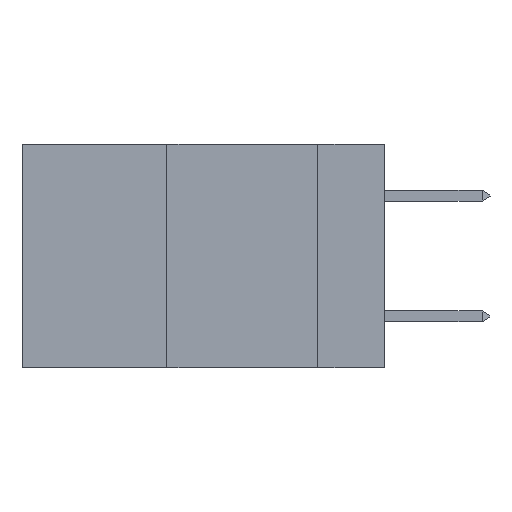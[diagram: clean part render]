
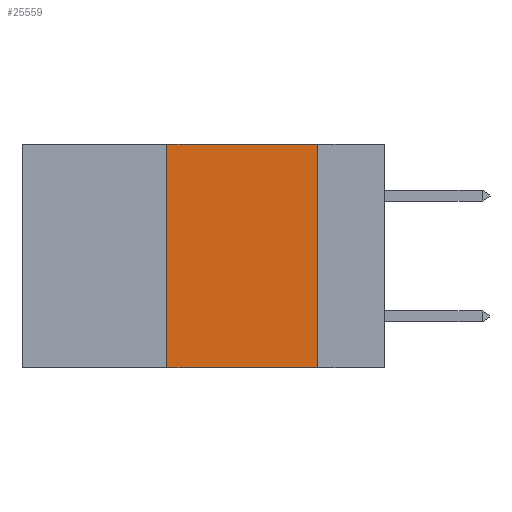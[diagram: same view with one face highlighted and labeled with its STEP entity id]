
A CAD part, left-side view. The second image highlights one B-rep face of the part: STEP entity #25559.
In plain terms, the highlighted planar face has unit normal (-1, 0, 0).
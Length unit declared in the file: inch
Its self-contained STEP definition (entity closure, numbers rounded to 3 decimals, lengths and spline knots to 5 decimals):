
#482 = CARTESIAN_POINT ( 'NONE',  ( 0., 0.6, 0. ) ) ;
#1963 = EDGE_LOOP ( 'NONE', ( #26776, #11105, #16997, #10084 ) ) ;
#3860 = LINE ( 'NONE', #15461, #24721 ) ;
#4085 = VERTEX_POINT ( 'NONE', #14336 ) ;
#4718 = DIRECTION ( 'NONE',  ( 0., 0., 1. ) ) ;
#6261 = LINE ( 'NONE', #32490, #35403 ) ;
#7123 = CARTESIAN_POINT ( 'NONE',  ( 0., 0.11, -0.37 ) ) ;
#7959 = CARTESIAN_POINT ( 'NONE',  ( 0., 0.6, 0. ) ) ;
#8156 = DIRECTION ( 'NONE',  ( 0., 0., -1. ) ) ;
#10084 = ORIENTED_EDGE ( 'NONE', *, *, #15928, .T. ) ;
#10442 = DIRECTION ( 'NONE',  ( 1., 0., 0. ) ) ;
#11105 = ORIENTED_EDGE ( 'NONE', *, *, #24320, .F. ) ;
#12488 = VECTOR ( 'NONE', #32417, 39.37008 ) ;
#13029 = VERTEX_POINT ( 'NONE', #32913 ) ;
#14336 = CARTESIAN_POINT ( 'NONE',  ( 0., 0.36, -0.37 ) ) ;
#15461 = CARTESIAN_POINT ( 'NONE',  ( 0., 0.11, 0. ) ) ;
#15928 = EDGE_CURVE ( 'NONE', #4085, #17012, #6261, .T. ) ;
#16038 = EDGE_CURVE ( 'NONE', #4085, #34879, #30956, .T. ) ;
#16997 = ORIENTED_EDGE ( 'NONE', *, *, #16038, .F. ) ;
#17012 = VERTEX_POINT ( 'NONE', #7123 ) ;
#19190 = FACE_OUTER_BOUND ( 'NONE', #1963, .T. ) ;
#21278 = CARTESIAN_POINT ( 'NONE',  ( 0., 0.36, 0. ) ) ;
#24134 = DIRECTION ( 'NONE',  ( 0., -1., 0. ) ) ;
#24320 = EDGE_CURVE ( 'NONE', #34879, #13029, #29759, .T. ) ;
#24721 = VECTOR ( 'NONE', #32192, 39.37008 ) ;
#25559 = ADVANCED_FACE ( 'NONE', ( #19190 ), #34376, .F. ) ;
#26229 = EDGE_CURVE ( 'NONE', #13029, #17012, #3860, .T. ) ;
#26776 = ORIENTED_EDGE ( 'NONE', *, *, #26229, .F. ) ;
#29759 = LINE ( 'NONE', #482, #12488 ) ;
#30591 = CARTESIAN_POINT ( 'NONE',  ( 0., 0.36, 0. ) ) ;
#30956 = LINE ( 'NONE', #30591, #34185 ) ;
#32192 = DIRECTION ( 'NONE',  ( 0., 0., -1. ) ) ;
#32417 = DIRECTION ( 'NONE',  ( 0., -1., 0. ) ) ;
#32490 = CARTESIAN_POINT ( 'NONE',  ( 0., 0.6, -0.37 ) ) ;
#32913 = CARTESIAN_POINT ( 'NONE',  ( 0., 0.11, 0. ) ) ;
#34185 = VECTOR ( 'NONE', #4718, 39.37008 ) ;
#34376 = PLANE ( 'NONE',  #36846 ) ;
#34879 = VERTEX_POINT ( 'NONE', #21278 ) ;
#35403 = VECTOR ( 'NONE', #24134, 39.37008 ) ;
#36846 = AXIS2_PLACEMENT_3D ( 'NONE', #7959, #10442, #8156 ) ;
